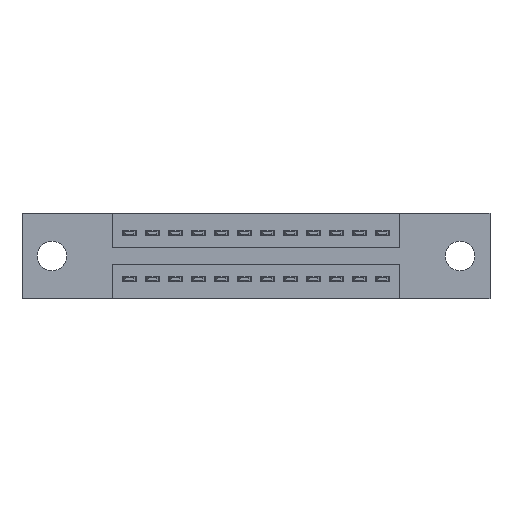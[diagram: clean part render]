
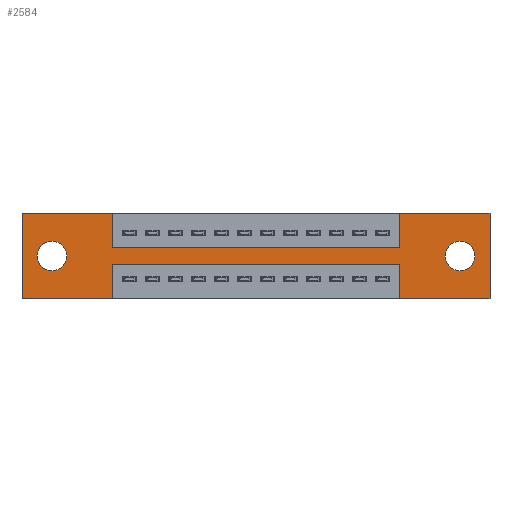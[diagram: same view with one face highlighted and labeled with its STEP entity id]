
A CAD part, front view. The second image highlights one B-rep face of the part: STEP entity #2584.
In plain terms, the highlighted planar face has unit normal (0, -1, 0).
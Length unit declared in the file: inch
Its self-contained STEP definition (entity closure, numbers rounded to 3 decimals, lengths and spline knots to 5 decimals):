
#110 = ORIENTED_EDGE ( 'NONE', *, *, #7106, .T. ) ;
#147 = CARTESIAN_POINT ( 'NONE',  ( 1.905, 0., -0.249 ) ) ;
#342 = CARTESIAN_POINT ( 'NONE',  ( 1.6425, 0., 0. ) ) ;
#402 = DIRECTION ( 'NONE',  ( 0., 0., -1. ) ) ;
#473 = VERTEX_POINT ( 'NONE', #4461 ) ;
#600 = VECTOR ( 'NONE', #4897, 39.37008 ) ;
#609 = AXIS2_PLACEMENT_3D ( 'NONE', #4660, #11728, #402 ) ;
#663 = ORIENTED_EDGE ( 'NONE', *, *, #7008, .F. ) ;
#690 = ORIENTED_EDGE ( 'NONE', *, *, #4469, .T. ) ;
#783 = EDGE_CURVE ( 'NONE', #6232, #4976, #3807, .T. ) ;
#943 = VECTOR ( 'NONE', #4070, 39.37008 ) ;
#1058 = AXIS2_PLACEMENT_3D ( 'NONE', #5013, #12162, #6031 ) ;
#1117 = DIRECTION ( 'NONE',  ( 0., 1., 0. ) ) ;
#1130 = DIRECTION ( 'NONE',  ( 1., 0., 0. ) ) ;
#1193 = DIRECTION ( 'NONE',  ( -1., 0., 0. ) ) ;
#1234 = LINE ( 'NONE', #13089, #600 ) ;
#1334 = DIRECTION ( 'NONE',  ( 0., 0., 1. ) ) ;
#1508 = ORIENTED_EDGE ( 'NONE', *, *, #9678, .F. ) ;
#1522 = ORIENTED_EDGE ( 'NONE', *, *, #4506, .F. ) ;
#1543 = VECTOR ( 'NONE', #11712, 39.37008 ) ;
#1570 = PLANE ( 'NONE',  #609 ) ;
#1677 = VERTEX_POINT ( 'NONE', #8145 ) ;
#1713 = ORIENTED_EDGE ( 'NONE', *, *, #6571, .F. ) ;
#1951 = EDGE_CURVE ( 'NONE', #7268, #6232, #7015, .T. ) ;
#1994 = ORIENTED_EDGE ( 'NONE', *, *, #2516, .F. ) ;
#2373 = CIRCLE ( 'NONE', #10337, 0.064 ) ;
#2466 = VECTOR ( 'NONE', #7157, 39.37008 ) ;
#2483 = LINE ( 'NONE', #8325, #10369 ) ;
#2516 = EDGE_CURVE ( 'NONE', #8047, #7871, #4685, .T. ) ;
#2584 = ADVANCED_FACE ( 'NONE', ( #6137, #9181, #4038 ), #1570, .T. ) ;
#3107 = CARTESIAN_POINT ( 'NONE',  ( 0.3925, 0., -0.15 ) ) ;
#3133 = CARTESIAN_POINT ( 'NONE',  ( 0., 0., 0. ) ) ;
#3172 = CARTESIAN_POINT ( 'NONE',  ( 2.035, 0., -0.37 ) ) ;
#3181 = DIRECTION ( 'NONE',  ( 0., 0., -1. ) ) ;
#3426 = ORIENTED_EDGE ( 'NONE', *, *, #8307, .F. ) ;
#3432 = LINE ( 'NONE', #6651, #6838 ) ;
#3502 = VERTEX_POINT ( 'NONE', #3172 ) ;
#3807 = LINE ( 'NONE', #3133, #5900 ) ;
#4026 = EDGE_CURVE ( 'NONE', #9065, #10126, #2373, .T. ) ;
#4038 = FACE_OUTER_BOUND ( 'NONE', #4567, .T. ) ;
#4070 = DIRECTION ( 'NONE',  ( 1., 0., 0. ) ) ;
#4246 = DIRECTION ( 'NONE',  ( 1., 0., 0. ) ) ;
#4261 = EDGE_CURVE ( 'NONE', #10116, #7252, #7374, .T. ) ;
#4461 = CARTESIAN_POINT ( 'NONE',  ( 1.905, 0., -0.121 ) ) ;
#4469 = EDGE_CURVE ( 'NONE', #473, #9621, #6879, .T. ) ;
#4506 = EDGE_CURVE ( 'NONE', #7871, #5146, #7998, .T. ) ;
#4567 = EDGE_LOOP ( 'NONE', ( #1713, #3426, #12669, #8966, #5370, #9460, #10269, #1508, #663, #1522, #1994, #6954 ) ) ;
#4579 = CIRCLE ( 'NONE', #8645, 0.064 ) ;
#4660 = CARTESIAN_POINT ( 'NONE',  ( 0., 0., -0.37 ) ) ;
#4685 = LINE ( 'NONE', #9592, #4839 ) ;
#4836 = CARTESIAN_POINT ( 'NONE',  ( 0.3925, 0., -0.22 ) ) ;
#4839 = VECTOR ( 'NONE', #11682, 39.37008 ) ;
#4897 = DIRECTION ( 'NONE',  ( 0., 0., -1. ) ) ;
#4976 = VERTEX_POINT ( 'NONE', #6873 ) ;
#5013 = CARTESIAN_POINT ( 'NONE',  ( 0.13, 0., -0.185 ) ) ;
#5085 = LINE ( 'NONE', #4836, #7638 ) ;
#5146 = VERTEX_POINT ( 'NONE', #7451 ) ;
#5221 = DIRECTION ( 'NONE',  ( 0., 1., 0. ) ) ;
#5240 = VECTOR ( 'NONE', #11146, 39.37008 ) ;
#5278 = VECTOR ( 'NONE', #4246, 39.37008 ) ;
#5356 = EDGE_CURVE ( 'NONE', #10126, #9065, #5724, .T. ) ;
#5370 = ORIENTED_EDGE ( 'NONE', *, *, #10224, .F. ) ;
#5724 = CIRCLE ( 'NONE', #1058, 0.064 ) ;
#5900 = VECTOR ( 'NONE', #1130, 39.37008 ) ;
#6031 = DIRECTION ( 'NONE',  ( 0., 0., 1. ) ) ;
#6048 = CARTESIAN_POINT ( 'NONE',  ( 0., 0., -0.37 ) ) ;
#6137 = FACE_BOUND ( 'NONE', #7954, .T. ) ;
#6232 = VERTEX_POINT ( 'NONE', #342 ) ;
#6260 = CARTESIAN_POINT ( 'NONE',  ( 0.3925, 0., -0.15 ) ) ;
#6418 = ORIENTED_EDGE ( 'NONE', *, *, #5356, .T. ) ;
#6513 = EDGE_CURVE ( 'NONE', #9957, #8047, #11317, .T. ) ;
#6571 = EDGE_CURVE ( 'NONE', #1677, #9957, #2483, .T. ) ;
#6651 = CARTESIAN_POINT ( 'NONE',  ( 0., 0., -0.37 ) ) ;
#6724 = VECTOR ( 'NONE', #1334, 39.37008 ) ;
#6838 = VECTOR ( 'NONE', #9722, 39.37008 ) ;
#6873 = CARTESIAN_POINT ( 'NONE',  ( 2.035, 0., 0. ) ) ;
#6879 = CIRCLE ( 'NONE', #7416, 0.064 ) ;
#6888 = LINE ( 'NONE', #6260, #5278 ) ;
#6954 = ORIENTED_EDGE ( 'NONE', *, *, #6513, .F. ) ;
#6996 = CARTESIAN_POINT ( 'NONE',  ( 0., 0., 0. ) ) ;
#7008 = EDGE_CURVE ( 'NONE', #5146, #13178, #12730, .T. ) ;
#7015 = LINE ( 'NONE', #12785, #1543 ) ;
#7106 = EDGE_CURVE ( 'NONE', #9621, #473, #4579, .T. ) ;
#7157 = DIRECTION ( 'NONE',  ( 0., 0., -1. ) ) ;
#7179 = DIRECTION ( 'NONE',  ( 0., 1., 0. ) ) ;
#7252 = VERTEX_POINT ( 'NONE', #8835 ) ;
#7268 = VERTEX_POINT ( 'NONE', #9761 ) ;
#7374 = LINE ( 'NONE', #10616, #6724 ) ;
#7416 = AXIS2_PLACEMENT_3D ( 'NONE', #10214, #7179, #8065 ) ;
#7449 = DIRECTION ( 'NONE',  ( 0., 0., 1. ) ) ;
#7451 = CARTESIAN_POINT ( 'NONE',  ( 0.3925, 0., 0. ) ) ;
#7528 = CARTESIAN_POINT ( 'NONE',  ( 1.6425, 0., -0.37 ) ) ;
#7638 = VECTOR ( 'NONE', #1193, 39.37008 ) ;
#7871 = VERTEX_POINT ( 'NONE', #8672 ) ;
#7954 = EDGE_LOOP ( 'NONE', ( #690, #110 ) ) ;
#7998 = LINE ( 'NONE', #6996, #943 ) ;
#8047 = VERTEX_POINT ( 'NONE', #13265 ) ;
#8065 = DIRECTION ( 'NONE',  ( 0., 0., -1. ) ) ;
#8144 = CARTESIAN_POINT ( 'NONE',  ( 0.3925, 0., -0.37 ) ) ;
#8145 = CARTESIAN_POINT ( 'NONE',  ( 0.3925, 0., -0.22 ) ) ;
#8307 = EDGE_CURVE ( 'NONE', #7252, #1677, #5085, .T. ) ;
#8325 = CARTESIAN_POINT ( 'NONE',  ( 0.3925, 0., -0.37 ) ) ;
#8486 = CARTESIAN_POINT ( 'NONE',  ( 1.905, 0., -0.185 ) ) ;
#8645 = AXIS2_PLACEMENT_3D ( 'NONE', #8486, #5221, #12361 ) ;
#8672 = CARTESIAN_POINT ( 'NONE',  ( 0., 0., 0. ) ) ;
#8835 = CARTESIAN_POINT ( 'NONE',  ( 1.6425, 0., -0.22 ) ) ;
#8966 = ORIENTED_EDGE ( 'NONE', *, *, #11381, .F. ) ;
#9065 = VERTEX_POINT ( 'NONE', #11147 ) ;
#9082 = EDGE_LOOP ( 'NONE', ( #10576, #6418 ) ) ;
#9181 = FACE_BOUND ( 'NONE', #9082, .T. ) ;
#9460 = ORIENTED_EDGE ( 'NONE', *, *, #783, .F. ) ;
#9592 = CARTESIAN_POINT ( 'NONE',  ( 0., 0., 0. ) ) ;
#9621 = VERTEX_POINT ( 'NONE', #147 ) ;
#9678 = EDGE_CURVE ( 'NONE', #13178, #7268, #6888, .T. ) ;
#9722 = DIRECTION ( 'NONE',  ( -1., 0., 0. ) ) ;
#9761 = CARTESIAN_POINT ( 'NONE',  ( 1.6425, 0., -0.15 ) ) ;
#9957 = VERTEX_POINT ( 'NONE', #8144 ) ;
#10116 = VERTEX_POINT ( 'NONE', #7528 ) ;
#10126 = VERTEX_POINT ( 'NONE', #11578 ) ;
#10214 = CARTESIAN_POINT ( 'NONE',  ( 1.905, 0., -0.185 ) ) ;
#10224 = EDGE_CURVE ( 'NONE', #4976, #3502, #1234, .T. ) ;
#10269 = ORIENTED_EDGE ( 'NONE', *, *, #1951, .F. ) ;
#10337 = AXIS2_PLACEMENT_3D ( 'NONE', #12442, #1117, #7449 ) ;
#10369 = VECTOR ( 'NONE', #3181, 39.37008 ) ;
#10576 = ORIENTED_EDGE ( 'NONE', *, *, #4026, .T. ) ;
#10616 = CARTESIAN_POINT ( 'NONE',  ( 1.6425, 0., -0.37 ) ) ;
#11146 = DIRECTION ( 'NONE',  ( -1., 0., 0. ) ) ;
#11147 = CARTESIAN_POINT ( 'NONE',  ( 0.13, 0., -0.121 ) ) ;
#11173 = CARTESIAN_POINT ( 'NONE',  ( 0.3925, 0., 0. ) ) ;
#11317 = LINE ( 'NONE', #6048, #5240 ) ;
#11381 = EDGE_CURVE ( 'NONE', #3502, #10116, #3432, .T. ) ;
#11578 = CARTESIAN_POINT ( 'NONE',  ( 0.13, 0., -0.249 ) ) ;
#11682 = DIRECTION ( 'NONE',  ( 0., 0., 1. ) ) ;
#11712 = DIRECTION ( 'NONE',  ( 0., 0., 1. ) ) ;
#11728 = DIRECTION ( 'NONE',  ( 0., -1., 0. ) ) ;
#12162 = DIRECTION ( 'NONE',  ( 0., 1., 0. ) ) ;
#12361 = DIRECTION ( 'NONE',  ( 0., 0., -1. ) ) ;
#12442 = CARTESIAN_POINT ( 'NONE',  ( 0.13, 0., -0.185 ) ) ;
#12669 = ORIENTED_EDGE ( 'NONE', *, *, #4261, .F. ) ;
#12730 = LINE ( 'NONE', #11173, #2466 ) ;
#12785 = CARTESIAN_POINT ( 'NONE',  ( 1.6425, 0., 0. ) ) ;
#13089 = CARTESIAN_POINT ( 'NONE',  ( 2.035, 0., 0. ) ) ;
#13178 = VERTEX_POINT ( 'NONE', #3107 ) ;
#13265 = CARTESIAN_POINT ( 'NONE',  ( 0., 0., -0.37 ) ) ;
